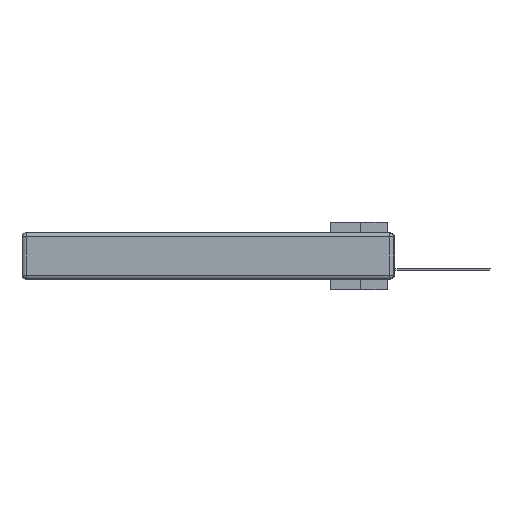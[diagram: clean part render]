
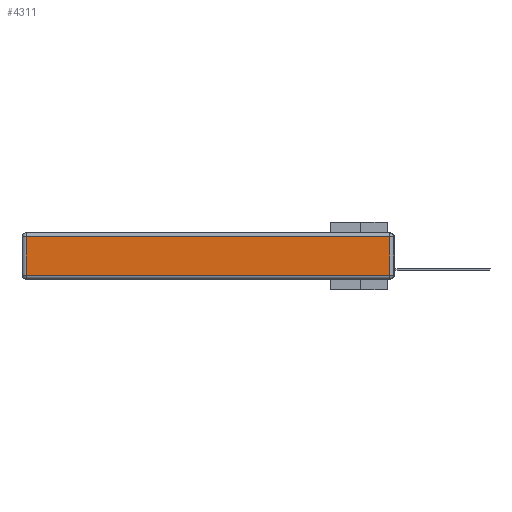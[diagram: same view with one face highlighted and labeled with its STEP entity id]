
A CAD part, left-side view. The second image highlights one B-rep face of the part: STEP entity #4311.
In plain terms, the highlighted planar face has unit normal (-1, 0, 0).
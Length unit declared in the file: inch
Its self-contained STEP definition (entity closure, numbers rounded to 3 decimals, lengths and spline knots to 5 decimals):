
#646 = VECTOR ( 'NONE', #1504, 39.37008 ) ;
#930 = LINE ( 'NONE', #27258, #646 ) ;
#1504 = DIRECTION ( 'NONE',  ( 0., 1., 0. ) ) ;
#2003 = VERTEX_POINT ( 'NONE', #6710 ) ;
#2093 = FACE_OUTER_BOUND ( 'NONE', #12085, .T. ) ;
#3530 = VERTEX_POINT ( 'NONE', #24153 ) ;
#3571 = ORIENTED_EDGE ( 'NONE', *, *, #20613, .T. ) ;
#4311 = ADVANCED_FACE ( 'NONE', ( #2093 ), #10859, .T. ) ;
#4411 = CARTESIAN_POINT ( 'NONE',  ( 0., 2.72, -0.343 ) ) ;
#4665 = DIRECTION ( 'NONE',  ( -1., 0., 0. ) ) ;
#4821 = CARTESIAN_POINT ( 'NONE',  ( 0., 0., -0.313 ) ) ;
#6168 = CARTESIAN_POINT ( 'NONE',  ( 0., 0.03, -0.313 ) ) ;
#6710 = CARTESIAN_POINT ( 'NONE',  ( 0., 2.72, -0.313 ) ) ;
#7816 = VECTOR ( 'NONE', #24943, 39.37008 ) ;
#7820 = ORIENTED_EDGE ( 'NONE', *, *, #9433, .T. ) ;
#8594 = VECTOR ( 'NONE', #11611, 39.37008 ) ;
#9433 = EDGE_CURVE ( 'NONE', #9843, #2003, #23707, .T. ) ;
#9780 = ORIENTED_EDGE ( 'NONE', *, *, #12157, .T. ) ;
#9843 = VERTEX_POINT ( 'NONE', #17034 ) ;
#10859 = PLANE ( 'NONE',  #20032 ) ;
#11611 = DIRECTION ( 'NONE',  ( 0., 0., 1. ) ) ;
#12085 = EDGE_LOOP ( 'NONE', ( #9780, #20957, #3571, #7820 ) ) ;
#12157 = EDGE_CURVE ( 'NONE', #2003, #14633, #22521, .T. ) ;
#14633 = VERTEX_POINT ( 'NONE', #6168 ) ;
#15440 = CARTESIAN_POINT ( 'NONE',  ( 0., 0., -0.343 ) ) ;
#17034 = CARTESIAN_POINT ( 'NONE',  ( 0., 2.72, -0.03 ) ) ;
#17478 = DIRECTION ( 'NONE',  ( 0., 0., -1. ) ) ;
#20032 = AXIS2_PLACEMENT_3D ( 'NONE', #15440, #4665, #26552 ) ;
#20613 = EDGE_CURVE ( 'NONE', #3530, #9843, #930, .T. ) ;
#20957 = ORIENTED_EDGE ( 'NONE', *, *, #26337, .T. ) ;
#21752 = VECTOR ( 'NONE', #17478, 39.37008 ) ;
#22521 = LINE ( 'NONE', #4821, #7816 ) ;
#23707 = LINE ( 'NONE', #4411, #21752 ) ;
#24153 = CARTESIAN_POINT ( 'NONE',  ( 0., 0.03, -0.03 ) ) ;
#24943 = DIRECTION ( 'NONE',  ( 0., -1., 0. ) ) ;
#26337 = EDGE_CURVE ( 'NONE', #14633, #3530, #26606, .T. ) ;
#26462 = CARTESIAN_POINT ( 'NONE',  ( 0., 0.03, -0.343 ) ) ;
#26552 = DIRECTION ( 'NONE',  ( 0., 0., 1. ) ) ;
#26606 = LINE ( 'NONE', #26462, #8594 ) ;
#27258 = CARTESIAN_POINT ( 'NONE',  ( 0., 2.75, -0.03 ) ) ;
